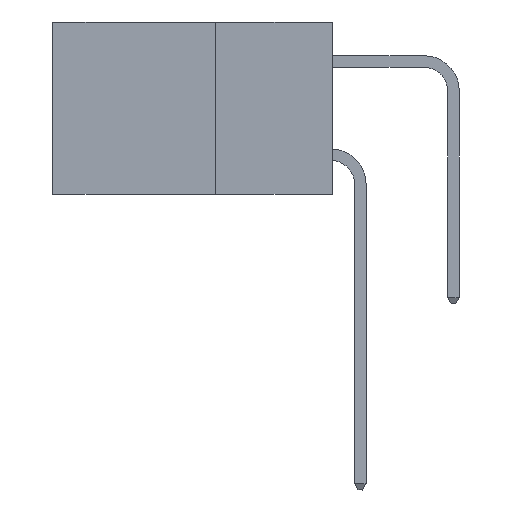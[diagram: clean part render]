
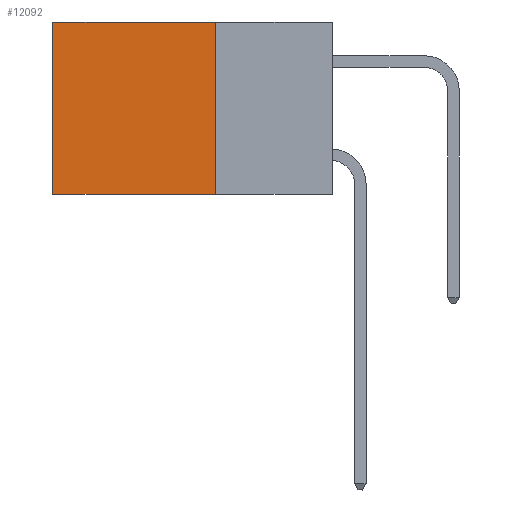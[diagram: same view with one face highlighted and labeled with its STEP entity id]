
A CAD part, left-side view. The second image highlights one B-rep face of the part: STEP entity #12092.
In plain terms, the highlighted planar face has unit normal (-1, 0, 0).
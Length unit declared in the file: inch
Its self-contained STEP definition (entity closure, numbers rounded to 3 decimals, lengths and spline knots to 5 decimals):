
#302 = CARTESIAN_POINT ( 'NONE',  ( 0.298, 0.6, 0. ) ) ;
#678 = VECTOR ( 'NONE', #16484, 39.37008 ) ;
#936 = ORIENTED_EDGE ( 'NONE', *, *, #2763, .T. ) ;
#977 = VECTOR ( 'NONE', #17121, 39.37008 ) ;
#1021 = ORIENTED_EDGE ( 'NONE', *, *, #2202, .T. ) ;
#2202 = EDGE_CURVE ( 'NONE', #15494, #12774, #9659, .T. ) ;
#2397 = VERTEX_POINT ( 'NONE', #13111 ) ;
#2763 = EDGE_CURVE ( 'NONE', #12774, #3609, #9421, .T. ) ;
#3609 = VERTEX_POINT ( 'NONE', #5162 ) ;
#4274 = LINE ( 'NONE', #8332, #678 ) ;
#4637 = DIRECTION ( 'NONE',  ( 0., 0., -1. ) ) ;
#4827 = DIRECTION ( 'NONE',  ( 1., 0., 0. ) ) ;
#5162 = CARTESIAN_POINT ( 'NONE',  ( 0.298, 0.6, -0.37 ) ) ;
#5173 = VECTOR ( 'NONE', #17153, 39.37008 ) ;
#5401 = CARTESIAN_POINT ( 'NONE',  ( 0.298, 0.25, 0. ) ) ;
#6196 = CARTESIAN_POINT ( 'NONE',  ( 0.298, 0.6, 0. ) ) ;
#6789 = FACE_OUTER_BOUND ( 'NONE', #15101, .T. ) ;
#7519 = PLANE ( 'NONE',  #17423 ) ;
#7562 = CARTESIAN_POINT ( 'NONE',  ( 0.298, 0.25, 0. ) ) ;
#8332 = CARTESIAN_POINT ( 'NONE',  ( 0.298, 0.25, -0.37 ) ) ;
#9421 = LINE ( 'NONE', #6196, #5173 ) ;
#9659 = LINE ( 'NONE', #11676, #977 ) ;
#10043 = ORIENTED_EDGE ( 'NONE', *, *, #14561, .F. ) ;
#10462 = EDGE_CURVE ( 'NONE', #2397, #3609, #4274, .T. ) ;
#11676 = CARTESIAN_POINT ( 'NONE',  ( 0.298, 0.25, 0. ) ) ;
#12092 = ADVANCED_FACE ( 'NONE', ( #6789 ), #7519, .F. ) ;
#12774 = VERTEX_POINT ( 'NONE', #302 ) ;
#12986 = CARTESIAN_POINT ( 'NONE',  ( 0.298, 0.25, 0. ) ) ;
#13111 = CARTESIAN_POINT ( 'NONE',  ( 0.298, 0.25, -0.37 ) ) ;
#13578 = VECTOR ( 'NONE', #4637, 39.37008 ) ;
#14419 = LINE ( 'NONE', #7562, #13578 ) ;
#14561 = EDGE_CURVE ( 'NONE', #15494, #2397, #14419, .T. ) ;
#15101 = EDGE_LOOP ( 'NONE', ( #936, #16329, #10043, #1021 ) ) ;
#15494 = VERTEX_POINT ( 'NONE', #5401 ) ;
#15698 = DIRECTION ( 'NONE',  ( 0., 0., -1. ) ) ;
#16329 = ORIENTED_EDGE ( 'NONE', *, *, #10462, .F. ) ;
#16484 = DIRECTION ( 'NONE',  ( 0., 1., 0. ) ) ;
#17121 = DIRECTION ( 'NONE',  ( 0., 1., 0. ) ) ;
#17153 = DIRECTION ( 'NONE',  ( 0., 0., -1. ) ) ;
#17423 = AXIS2_PLACEMENT_3D ( 'NONE', #12986, #4827, #15698 ) ;
